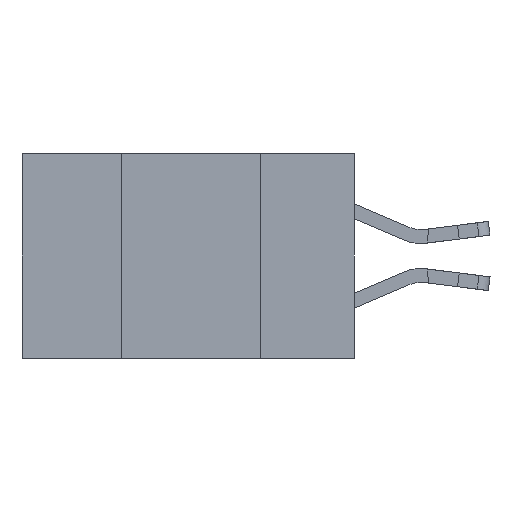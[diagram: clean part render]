
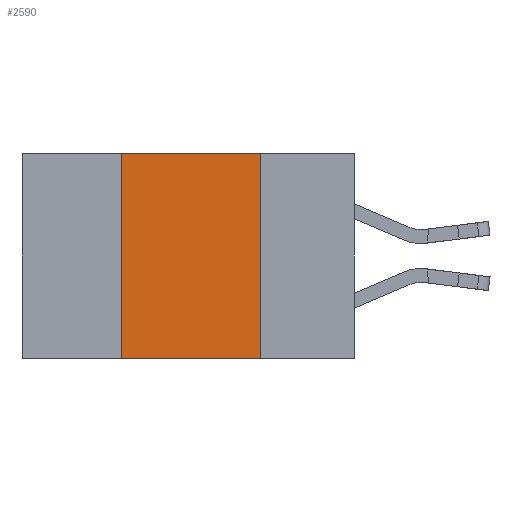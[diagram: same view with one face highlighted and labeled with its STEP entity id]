
A CAD part, left-side view. The second image highlights one B-rep face of the part: STEP entity #2590.
In plain terms, the highlighted planar face has unit normal (-1, 0, 0).
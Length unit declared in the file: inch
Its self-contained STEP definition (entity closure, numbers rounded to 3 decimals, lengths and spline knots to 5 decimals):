
#429 = VERTEX_POINT ( 'NONE', #3218 ) ;
#795 = DIRECTION ( 'NONE',  ( 0., 0., -1. ) ) ;
#847 = CARTESIAN_POINT ( 'NONE',  ( 0., 0.42, -0.37 ) ) ;
#1461 = LINE ( 'NONE', #2696, #10839 ) ;
#1485 = DIRECTION ( 'NONE',  ( 0., 0., -1. ) ) ;
#1667 = ORIENTED_EDGE ( 'NONE', *, *, #6331, .F. ) ;
#1750 = CARTESIAN_POINT ( 'NONE',  ( 0., 0.42, 0. ) ) ;
#2590 = ADVANCED_FACE ( 'NONE', ( #7821 ), #6389, .F. ) ;
#2696 = CARTESIAN_POINT ( 'NONE',  ( 0., 0.6, -0.37 ) ) ;
#3115 = EDGE_CURVE ( 'NONE', #7141, #11111, #1461, .T. ) ;
#3218 = CARTESIAN_POINT ( 'NONE',  ( 0., 0.17, 0. ) ) ;
#3971 = ORIENTED_EDGE ( 'NONE', *, *, #10736, .F. ) ;
#4151 = AXIS2_PLACEMENT_3D ( 'NONE', #5281, #6184, #795 ) ;
#5281 = CARTESIAN_POINT ( 'NONE',  ( 0., 0.6, 0. ) ) ;
#5360 = VECTOR ( 'NONE', #8016, 39.37008 ) ;
#5758 = EDGE_LOOP ( 'NONE', ( #1667, #3971, #11249, #11421 ) ) ;
#5967 = VECTOR ( 'NONE', #1485, 39.37008 ) ;
#6184 = DIRECTION ( 'NONE',  ( 1., 0., 0. ) ) ;
#6331 = EDGE_CURVE ( 'NONE', #429, #11111, #7282, .T. ) ;
#6389 = PLANE ( 'NONE',  #4151 ) ;
#7141 = VERTEX_POINT ( 'NONE', #10400 ) ;
#7282 = LINE ( 'NONE', #9682, #5967 ) ;
#7821 = FACE_OUTER_BOUND ( 'NONE', #5758, .T. ) ;
#8016 = DIRECTION ( 'NONE',  ( 0., 0., 1. ) ) ;
#8083 = EDGE_CURVE ( 'NONE', #7141, #8909, #9224, .T. ) ;
#8909 = VERTEX_POINT ( 'NONE', #1750 ) ;
#8986 = CARTESIAN_POINT ( 'NONE',  ( 0., 0.6, 0. ) ) ;
#9224 = LINE ( 'NONE', #847, #5360 ) ;
#9538 = VECTOR ( 'NONE', #10852, 39.37008 ) ;
#9682 = CARTESIAN_POINT ( 'NONE',  ( 0., 0.17, -0.37 ) ) ;
#9823 = DIRECTION ( 'NONE',  ( 0., -1., 0. ) ) ;
#10020 = CARTESIAN_POINT ( 'NONE',  ( 0., 0.17, -0.37 ) ) ;
#10400 = CARTESIAN_POINT ( 'NONE',  ( 0., 0.42, -0.37 ) ) ;
#10736 = EDGE_CURVE ( 'NONE', #8909, #429, #10959, .T. ) ;
#10839 = VECTOR ( 'NONE', #9823, 39.37008 ) ;
#10852 = DIRECTION ( 'NONE',  ( 0., -1., 0. ) ) ;
#10959 = LINE ( 'NONE', #8986, #9538 ) ;
#11111 = VERTEX_POINT ( 'NONE', #10020 ) ;
#11249 = ORIENTED_EDGE ( 'NONE', *, *, #8083, .F. ) ;
#11421 = ORIENTED_EDGE ( 'NONE', *, *, #3115, .T. ) ;
